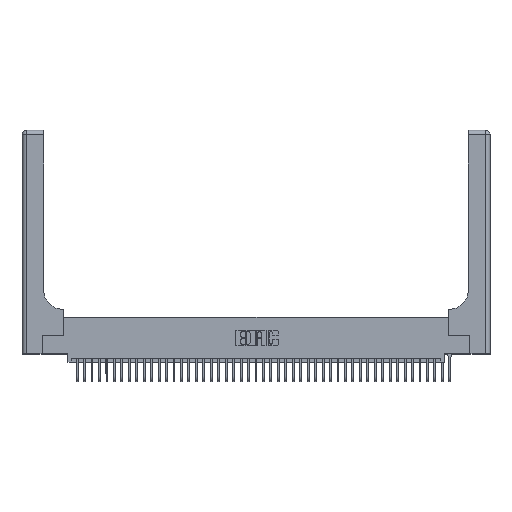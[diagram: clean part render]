
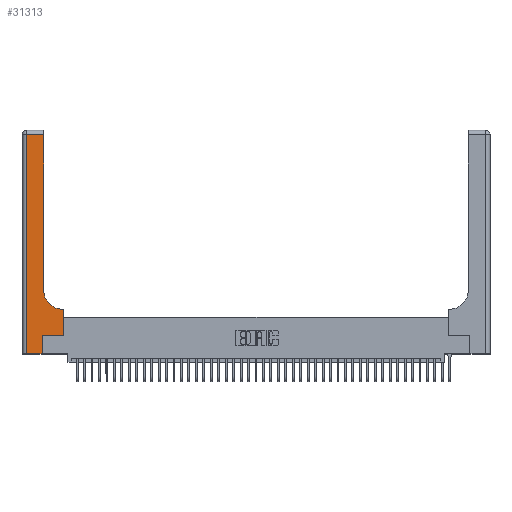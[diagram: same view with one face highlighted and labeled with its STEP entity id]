
A CAD part, top view. The second image highlights one B-rep face of the part: STEP entity #31313.
In plain terms, the highlighted planar face has unit normal (0, 0, 1).
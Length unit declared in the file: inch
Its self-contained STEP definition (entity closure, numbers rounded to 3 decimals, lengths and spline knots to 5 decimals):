
#95 = VECTOR ( 'NONE', #2447, 39.37008 ) ;
#583 = CARTESIAN_POINT ( 'NONE',  ( 0.2915, 0.6, 0.37 ) ) ;
#723 = LINE ( 'NONE', #39905, #18950 ) ;
#740 = ORIENTED_EDGE ( 'NONE', *, *, #12261, .T. ) ;
#939 = CARTESIAN_POINT ( 'NONE',  ( 0., 0., 0.37 ) ) ;
#1251 = EDGE_CURVE ( 'NONE', #2650, #24860, #16422, .T. ) ;
#1916 = ORIENTED_EDGE ( 'NONE', *, *, #26860, .T. ) ;
#2447 = DIRECTION ( 'NONE',  ( 0., 1., 0. ) ) ;
#2650 = VERTEX_POINT ( 'NONE', #15838 ) ;
#2700 = PLANE ( 'NONE',  #28594 ) ;
#3017 = CARTESIAN_POINT ( 'NONE',  ( 0.2915, 0.85, 0.37 ) ) ;
#3311 = VERTEX_POINT ( 'NONE', #26243 ) ;
#3423 = DIRECTION ( 'NONE',  ( 0., 1., 0. ) ) ;
#3452 = CARTESIAN_POINT ( 'NONE',  ( 0.2915, 2.94, 0.37 ) ) ;
#4169 = LINE ( 'NONE', #28435, #12844 ) ;
#4297 = AXIS2_PLACEMENT_3D ( 'NONE', #15267, #37468, #18494 ) ;
#5702 = CARTESIAN_POINT ( 'NONE',  ( 0.269, 0., 0.37 ) ) ;
#5826 = EDGE_LOOP ( 'NONE', ( #1916, #12084, #12642, #39931, #18512, #740, #32314, #32109, #8422 ) ) ;
#5972 = DIRECTION ( 'NONE',  ( 0., 0., -1. ) ) ;
#6175 = LINE ( 'NONE', #583, #39116 ) ;
#7247 = VERTEX_POINT ( 'NONE', #23097 ) ;
#8126 = EDGE_CURVE ( 'NONE', #34165, #3311, #723, .T. ) ;
#8311 = LINE ( 'NONE', #37297, #41097 ) ;
#8422 = ORIENTED_EDGE ( 'NONE', *, *, #1251, .T. ) ;
#8797 = LINE ( 'NONE', #5702, #95 ) ;
#10014 = VECTOR ( 'NONE', #3423, 39.37008 ) ;
#12084 = ORIENTED_EDGE ( 'NONE', *, *, #29231, .T. ) ;
#12152 = EDGE_CURVE ( 'NONE', #7247, #22088, #8311, .T. ) ;
#12261 = EDGE_CURVE ( 'NONE', #21809, #34165, #4169, .T. ) ;
#12398 = CARTESIAN_POINT ( 'NONE',  ( 0., 3., 0.37 ) ) ;
#12642 = ORIENTED_EDGE ( 'NONE', *, *, #12152, .T. ) ;
#12844 = VECTOR ( 'NONE', #40968, 39.37008 ) ;
#13025 = EDGE_CURVE ( 'NONE', #30301, #21809, #8797, .T. ) ;
#13325 = EDGE_CURVE ( 'NONE', #3311, #2650, #6175, .T. ) ;
#13618 = CARTESIAN_POINT ( 'NONE',  ( 0.269, 0., 0.37 ) ) ;
#14059 = VECTOR ( 'NONE', #32886, 39.37008 ) ;
#15267 = CARTESIAN_POINT ( 'NONE',  ( 0.5415, 0.85, 0.37 ) ) ;
#15838 = CARTESIAN_POINT ( 'NONE',  ( 0.5415, 0.6, 0.37 ) ) ;
#16422 = CIRCLE ( 'NONE', #4297, 0.25 ) ;
#16454 = CARTESIAN_POINT ( 'NONE',  ( 0.2915, 3., 0.37 ) ) ;
#16855 = DIRECTION ( 'NONE',  ( -1., 0., 0. ) ) ;
#18494 = DIRECTION ( 'NONE',  ( 1., 0., 0. ) ) ;
#18512 = ORIENTED_EDGE ( 'NONE', *, *, #13025, .T. ) ;
#18950 = VECTOR ( 'NONE', #20804, 39.37008 ) ;
#19776 = CARTESIAN_POINT ( 'NONE',  ( 0.06, 0., 0.37 ) ) ;
#20804 = DIRECTION ( 'NONE',  ( 0., 1., 0. ) ) ;
#21809 = VERTEX_POINT ( 'NONE', #31194 ) ;
#22088 = VERTEX_POINT ( 'NONE', #19776 ) ;
#23097 = CARTESIAN_POINT ( 'NONE',  ( 0.06, 2.94, 0.37 ) ) ;
#24551 = LINE ( 'NONE', #939, #14059 ) ;
#24740 = DIRECTION ( 'NONE',  ( 0., -1., 0. ) ) ;
#24860 = VERTEX_POINT ( 'NONE', #3017 ) ;
#26243 = CARTESIAN_POINT ( 'NONE',  ( 0.5585, 0.6, 0.37 ) ) ;
#26860 = EDGE_CURVE ( 'NONE', #24860, #38139, #34447, .T. ) ;
#27822 = VECTOR ( 'NONE', #40613, 39.37008 ) ;
#28407 = DIRECTION ( 'NONE',  ( -1., 0., 0. ) ) ;
#28435 = CARTESIAN_POINT ( 'NONE',  ( 0.269, 0.25, 0.37 ) ) ;
#28594 = AXIS2_PLACEMENT_3D ( 'NONE', #12398, #5972, #28407 ) ;
#28652 = FACE_OUTER_BOUND ( 'NONE', #5826, .T. ) ;
#29231 = EDGE_CURVE ( 'NONE', #38139, #7247, #34289, .T. ) ;
#30301 = VERTEX_POINT ( 'NONE', #13618 ) ;
#31194 = CARTESIAN_POINT ( 'NONE',  ( 0.269, 0.25, 0.37 ) ) ;
#31313 = ADVANCED_FACE ( 'NONE', ( #28652 ), #2700, .F. ) ;
#32109 = ORIENTED_EDGE ( 'NONE', *, *, #13325, .T. ) ;
#32314 = ORIENTED_EDGE ( 'NONE', *, *, #8126, .T. ) ;
#32886 = DIRECTION ( 'NONE',  ( 1., 0., 0. ) ) ;
#34165 = VERTEX_POINT ( 'NONE', #38874 ) ;
#34289 = LINE ( 'NONE', #40747, #27822 ) ;
#34447 = LINE ( 'NONE', #16454, #10014 ) ;
#37297 = CARTESIAN_POINT ( 'NONE',  ( 0.06, 3., 0.37 ) ) ;
#37468 = DIRECTION ( 'NONE',  ( 0., 0., -1. ) ) ;
#37760 = EDGE_CURVE ( 'NONE', #22088, #30301, #24551, .T. ) ;
#38139 = VERTEX_POINT ( 'NONE', #3452 ) ;
#38874 = CARTESIAN_POINT ( 'NONE',  ( 0.5585, 0.25, 0.37 ) ) ;
#39116 = VECTOR ( 'NONE', #16855, 39.37008 ) ;
#39905 = CARTESIAN_POINT ( 'NONE',  ( 0.5585, 0.25, 0.37 ) ) ;
#39931 = ORIENTED_EDGE ( 'NONE', *, *, #37760, .T. ) ;
#40613 = DIRECTION ( 'NONE',  ( -1., 0., 0. ) ) ;
#40747 = CARTESIAN_POINT ( 'NONE',  ( 0., 2.94, 0.37 ) ) ;
#40968 = DIRECTION ( 'NONE',  ( 1., 0., 0. ) ) ;
#41097 = VECTOR ( 'NONE', #24740, 39.37008 ) ;
